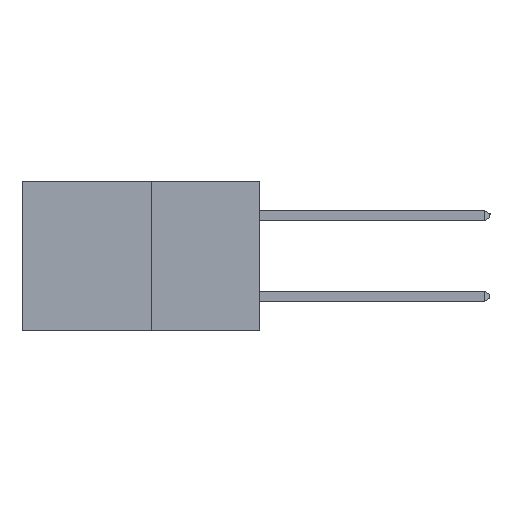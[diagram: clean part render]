
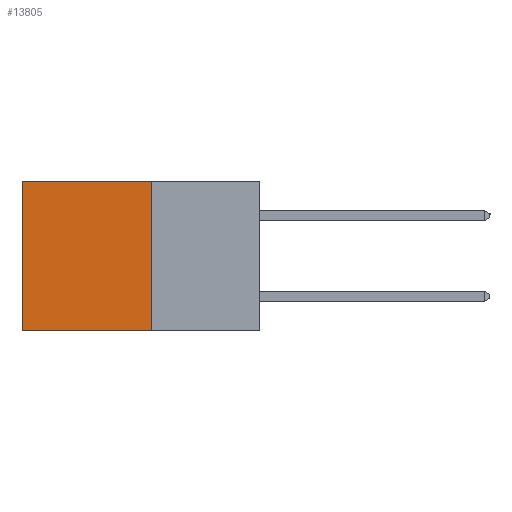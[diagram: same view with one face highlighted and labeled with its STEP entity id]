
A CAD part, left-side view. The second image highlights one B-rep face of the part: STEP entity #13805.
In plain terms, the highlighted planar face has unit normal (-1, 0, 0).
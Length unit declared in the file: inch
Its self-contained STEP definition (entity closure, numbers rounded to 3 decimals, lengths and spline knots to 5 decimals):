
#116 = LINE ( 'NONE', #1246, #11092 ) ;
#262 = VERTEX_POINT ( 'NONE', #7775 ) ;
#661 = FACE_OUTER_BOUND ( 'NONE', #14022, .T. ) ;
#1059 = ORIENTED_EDGE ( 'NONE', *, *, #13043, .T. ) ;
#1194 = ORIENTED_EDGE ( 'NONE', *, *, #9627, .F. ) ;
#1246 = CARTESIAN_POINT ( 'NONE',  ( 0.277, 0.27, -0.37 ) ) ;
#1280 = DIRECTION ( 'NONE',  ( 0., 1., 0. ) ) ;
#1475 = VERTEX_POINT ( 'NONE', #5099 ) ;
#1568 = PLANE ( 'NONE',  #2890 ) ;
#1801 = CARTESIAN_POINT ( 'NONE',  ( 0.277, 0.59, -0.37 ) ) ;
#2188 = CARTESIAN_POINT ( 'NONE',  ( 0.277, 0.27, 0. ) ) ;
#2594 = CARTESIAN_POINT ( 'NONE',  ( 0.277, 0.27, -0.37 ) ) ;
#2638 = DIRECTION ( 'NONE',  ( 0., 0., -1. ) ) ;
#2890 = AXIS2_PLACEMENT_3D ( 'NONE', #2594, #9309, #2638 ) ;
#4247 = ORIENTED_EDGE ( 'NONE', *, *, #11002, .T. ) ;
#4397 = LINE ( 'NONE', #2188, #7405 ) ;
#5099 = CARTESIAN_POINT ( 'NONE',  ( 0.277, 0.27, 0. ) ) ;
#6025 = VECTOR ( 'NONE', #13632, 39.37008 ) ;
#6075 = CARTESIAN_POINT ( 'NONE',  ( 0.277, 0.27, -0.37 ) ) ;
#6189 = VERTEX_POINT ( 'NONE', #12244 ) ;
#6309 = EDGE_CURVE ( 'NONE', #262, #13945, #116, .T. ) ;
#7128 = VECTOR ( 'NONE', #13064, 39.37008 ) ;
#7405 = VECTOR ( 'NONE', #13061, 39.37008 ) ;
#7462 = LINE ( 'NONE', #11984, #7128 ) ;
#7775 = CARTESIAN_POINT ( 'NONE',  ( 0.277, 0.27, -0.37 ) ) ;
#9309 = DIRECTION ( 'NONE',  ( 1., 0., 0. ) ) ;
#9627 = EDGE_CURVE ( 'NONE', #1475, #262, #11807, .T. ) ;
#11002 = EDGE_CURVE ( 'NONE', #6189, #13945, #7462, .T. ) ;
#11092 = VECTOR ( 'NONE', #1280, 39.37008 ) ;
#11807 = LINE ( 'NONE', #6075, #6025 ) ;
#11984 = CARTESIAN_POINT ( 'NONE',  ( 0.277, 0.59, -0.37 ) ) ;
#12244 = CARTESIAN_POINT ( 'NONE',  ( 0.277, 0.59, 0. ) ) ;
#13043 = EDGE_CURVE ( 'NONE', #1475, #6189, #4397, .T. ) ;
#13061 = DIRECTION ( 'NONE',  ( 0., 1., 0. ) ) ;
#13064 = DIRECTION ( 'NONE',  ( 0., 0., -1. ) ) ;
#13537 = ORIENTED_EDGE ( 'NONE', *, *, #6309, .F. ) ;
#13632 = DIRECTION ( 'NONE',  ( 0., 0., -1. ) ) ;
#13805 = ADVANCED_FACE ( 'NONE', ( #661 ), #1568, .F. ) ;
#13945 = VERTEX_POINT ( 'NONE', #1801 ) ;
#14022 = EDGE_LOOP ( 'NONE', ( #4247, #13537, #1194, #1059 ) ) ;
